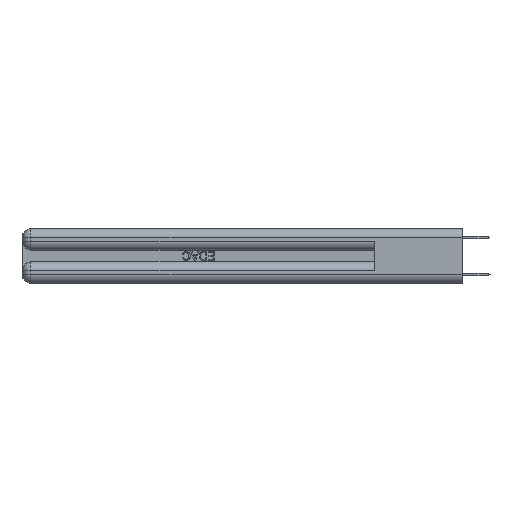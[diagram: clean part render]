
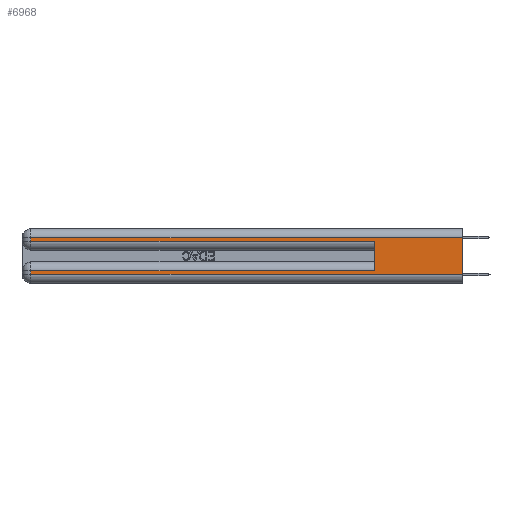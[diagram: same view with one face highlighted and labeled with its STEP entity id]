
A CAD part, left-side view. The second image highlights one B-rep face of the part: STEP entity #6968.
In plain terms, the highlighted planar face has unit normal (-1, 0, 0).
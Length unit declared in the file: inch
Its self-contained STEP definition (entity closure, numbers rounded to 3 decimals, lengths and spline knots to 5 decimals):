
#283 = VECTOR ( 'NONE', #10829, 39.37008 ) ;
#406 = CARTESIAN_POINT ( 'NONE',  ( 0., 0., 0.06 ) ) ;
#1988 = DIRECTION ( 'NONE',  ( 0., 0., -1. ) ) ;
#2093 = LINE ( 'NONE', #32960, #22395 ) ;
#2105 = EDGE_CURVE ( 'NONE', #5408, #15090, #2093, .T. ) ;
#2150 = VECTOR ( 'NONE', #21054, 39.37008 ) ;
#2820 = VERTEX_POINT ( 'NONE', #6393 ) ;
#2846 = CARTESIAN_POINT ( 'NONE',  ( 0., 0.6, 0.285 ) ) ;
#2937 = CARTESIAN_POINT ( 'NONE',  ( 0., 2.94, 0.285 ) ) ;
#4360 = CARTESIAN_POINT ( 'NONE',  ( 0., 0., 0.37 ) ) ;
#5089 = DIRECTION ( 'NONE',  ( 0., -1., 0. ) ) ;
#5408 = VERTEX_POINT ( 'NONE', #30469 ) ;
#5435 = VERTEX_POINT ( 'NONE', #32925 ) ;
#6324 = LINE ( 'NONE', #8584, #2150 ) ;
#6393 = CARTESIAN_POINT ( 'NONE',  ( 0., 2.94, 0.085 ) ) ;
#6968 = ADVANCED_FACE ( 'NONE', ( #33171 ), #7091, .F. ) ;
#7091 = PLANE ( 'NONE',  #28006 ) ;
#7602 = LINE ( 'NONE', #4360, #18594 ) ;
#7627 = EDGE_LOOP ( 'NONE', ( #23415, #26273, #14000, #35486, #25706, #23650, #35279, #16014 ) ) ;
#8584 = CARTESIAN_POINT ( 'NONE',  ( 0., 0.6, 0.145 ) ) ;
#9037 = VERTEX_POINT ( 'NONE', #406 ) ;
#9984 = LINE ( 'NONE', #33611, #36588 ) ;
#10427 = DIRECTION ( 'NONE',  ( 0., 0., -1. ) ) ;
#10740 = DIRECTION ( 'NONE',  ( 0., 1., 0. ) ) ;
#10829 = DIRECTION ( 'NONE',  ( 0., -1., 0. ) ) ;
#11197 = CARTESIAN_POINT ( 'NONE',  ( 0., 0.6, 0.085 ) ) ;
#12440 = EDGE_CURVE ( 'NONE', #20891, #9037, #33517, .T. ) ;
#13145 = CARTESIAN_POINT ( 'NONE',  ( 0., 2.94, 0.06 ) ) ;
#14000 = ORIENTED_EDGE ( 'NONE', *, *, #2105, .T. ) ;
#14588 = LINE ( 'NONE', #29684, #20467 ) ;
#14661 = EDGE_CURVE ( 'NONE', #5435, #5408, #37238, .T. ) ;
#14899 = VECTOR ( 'NONE', #5089, 39.37008 ) ;
#15090 = VERTEX_POINT ( 'NONE', #2937 ) ;
#15800 = VERTEX_POINT ( 'NONE', #2846 ) ;
#16014 = ORIENTED_EDGE ( 'NONE', *, *, #12440, .T. ) ;
#16962 = VERTEX_POINT ( 'NONE', #11197 ) ;
#18594 = VECTOR ( 'NONE', #10427, 39.37008 ) ;
#19497 = LINE ( 'NONE', #31003, #14899 ) ;
#20467 = VECTOR ( 'NONE', #31779, 39.37008 ) ;
#20891 = VERTEX_POINT ( 'NONE', #13145 ) ;
#21054 = DIRECTION ( 'NONE',  ( 0., 0., 1. ) ) ;
#21248 = EDGE_CURVE ( 'NONE', #16962, #15800, #6324, .T. ) ;
#22335 = CARTESIAN_POINT ( 'NONE',  ( 0., 0., 0.31 ) ) ;
#22357 = EDGE_CURVE ( 'NONE', #16962, #2820, #9984, .T. ) ;
#22395 = VECTOR ( 'NONE', #24260, 39.37008 ) ;
#23415 = ORIENTED_EDGE ( 'NONE', *, *, #24142, .F. ) ;
#23650 = ORIENTED_EDGE ( 'NONE', *, *, #22357, .T. ) ;
#24142 = EDGE_CURVE ( 'NONE', #5435, #9037, #7602, .T. ) ;
#24260 = DIRECTION ( 'NONE',  ( 0., 0., -1. ) ) ;
#25706 = ORIENTED_EDGE ( 'NONE', *, *, #21248, .F. ) ;
#25732 = EDGE_CURVE ( 'NONE', #2820, #20891, #14588, .T. ) ;
#26273 = ORIENTED_EDGE ( 'NONE', *, *, #14661, .T. ) ;
#28006 = AXIS2_PLACEMENT_3D ( 'NONE', #35994, #28078, #1988 ) ;
#28078 = DIRECTION ( 'NONE',  ( 1., 0., 0. ) ) ;
#29684 = CARTESIAN_POINT ( 'NONE',  ( 0., 2.94, 0.37 ) ) ;
#30469 = CARTESIAN_POINT ( 'NONE',  ( 0., 2.94, 0.31 ) ) ;
#31003 = CARTESIAN_POINT ( 'NONE',  ( 0., 0., 0.285 ) ) ;
#31766 = DIRECTION ( 'NONE',  ( 0., 1., 0. ) ) ;
#31779 = DIRECTION ( 'NONE',  ( 0., 0., -1. ) ) ;
#32091 = VECTOR ( 'NONE', #31766, 39.37008 ) ;
#32925 = CARTESIAN_POINT ( 'NONE',  ( 0., 0., 0.31 ) ) ;
#32960 = CARTESIAN_POINT ( 'NONE',  ( 0., 2.94, 0.37 ) ) ;
#33171 = FACE_OUTER_BOUND ( 'NONE', #7627, .T. ) ;
#33517 = LINE ( 'NONE', #36705, #283 ) ;
#33611 = CARTESIAN_POINT ( 'NONE',  ( 0., 0., 0.085 ) ) ;
#34594 = EDGE_CURVE ( 'NONE', #15090, #15800, #19497, .T. ) ;
#35279 = ORIENTED_EDGE ( 'NONE', *, *, #25732, .T. ) ;
#35486 = ORIENTED_EDGE ( 'NONE', *, *, #34594, .T. ) ;
#35994 = CARTESIAN_POINT ( 'NONE',  ( 0., 0., 0.37 ) ) ;
#36588 = VECTOR ( 'NONE', #10740, 39.37008 ) ;
#36705 = CARTESIAN_POINT ( 'NONE',  ( 0., 0., 0.06 ) ) ;
#37238 = LINE ( 'NONE', #22335, #32091 ) ;
